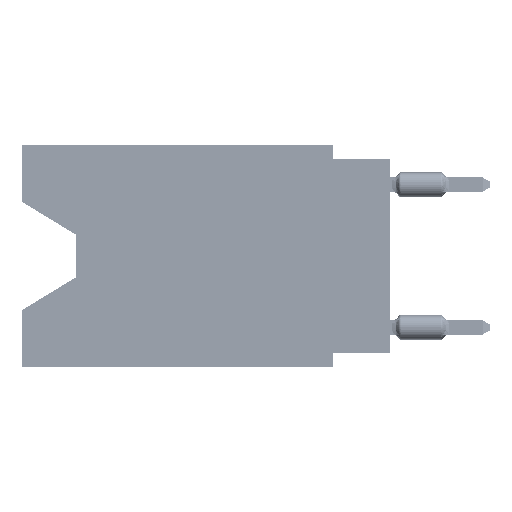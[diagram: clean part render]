
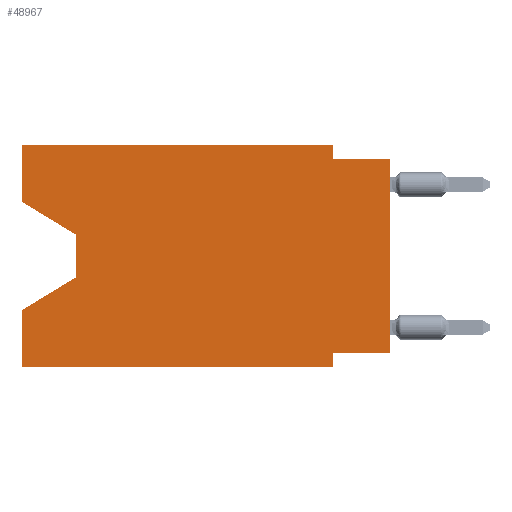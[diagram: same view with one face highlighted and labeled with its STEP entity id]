
A CAD part, left-side view. The second image highlights one B-rep face of the part: STEP entity #48967.
In plain terms, the highlighted planar face has unit normal (-1, 0, 0).
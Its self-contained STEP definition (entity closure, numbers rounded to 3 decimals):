
#384 = EDGE_CURVE ( 'NONE', #65976, #65730, #19403, .T. ) ;
#925 = DIRECTION ( 'NONE',  ( 0., 0., 1. ) ) ;
#1630 = LINE ( 'NONE', #21881, #24821 ) ;
#2386 = ORIENTED_EDGE ( 'NONE', *, *, #59878, .F. ) ;
#3034 = EDGE_CURVE ( 'NONE', #25149, #25658, #43328, .T. ) ;
#4413 = CARTESIAN_POINT ( 'NONE',  ( 0., 16.383, -2.546 ) ) ;
#4581 = LINE ( 'NONE', #29828, #42980 ) ;
#5209 = VECTOR ( 'NONE', #25772, 1000. ) ;
#5611 = ORIENTED_EDGE ( 'NONE', *, *, #67015, .T. ) ;
#5755 = ORIENTED_EDGE ( 'NONE', *, *, #31479, .T. ) ;
#6638 = DIRECTION ( 'NONE',  ( 0., 0., -1. ) ) ;
#7127 = CARTESIAN_POINT ( 'NONE',  ( 0., 16.383, 0. ) ) ;
#7398 = ORIENTED_EDGE ( 'NONE', *, *, #20779, .F. ) ;
#9012 = VECTOR ( 'NONE', #29180, 1000. ) ;
#9027 = ORIENTED_EDGE ( 'NONE', *, *, #65738, .F. ) ;
#9555 = DIRECTION ( 'NONE',  ( 0., -1., 0. ) ) ;
#11085 = VECTOR ( 'NONE', #25171, 1000. ) ;
#13468 = EDGE_LOOP ( 'NONE', ( #39283, #5611, #14471, #36393, #50092, #57030, #2386, #5755, #9027, #33140, #7398, #24245 ) ) ;
#14422 = CARTESIAN_POINT ( 'NONE',  ( 0., 16.383, -9.906 ) ) ;
#14471 = ORIENTED_EDGE ( 'NONE', *, *, #19290, .T. ) ;
#15254 = AXIS2_PLACEMENT_3D ( 'NONE', #66269, #39797, #47651 ) ;
#15755 = CARTESIAN_POINT ( 'NONE',  ( 0., 13.97, -4.013 ) ) ;
#19283 = VECTOR ( 'NONE', #70309, 1000. ) ;
#19290 = EDGE_CURVE ( 'NONE', #57836, #50094, #39008, .T. ) ;
#19403 = LINE ( 'NONE', #20606, #19283 ) ;
#20059 = CARTESIAN_POINT ( 'NONE',  ( 0., 16.383, 0. ) ) ;
#20606 = CARTESIAN_POINT ( 'NONE',  ( 0., 16.383, -9.906 ) ) ;
#20779 = EDGE_CURVE ( 'NONE', #68267, #77958, #39117, .T. ) ;
#21881 = CARTESIAN_POINT ( 'NONE',  ( 0., 2.54, 0. ) ) ;
#24180 = CARTESIAN_POINT ( 'NONE',  ( 0., 2.54, -9.906 ) ) ;
#24245 = ORIENTED_EDGE ( 'NONE', *, *, #66612, .F. ) ;
#24821 = VECTOR ( 'NONE', #40944, 1000. ) ;
#25149 = VERTEX_POINT ( 'NONE', #68659 ) ;
#25171 = DIRECTION ( 'NONE',  ( 0., 0., 1. ) ) ;
#25658 = VERTEX_POINT ( 'NONE', #15755 ) ;
#25772 = DIRECTION ( 'NONE',  ( 0., 0.855, -0.519 ) ) ;
#26176 = CARTESIAN_POINT ( 'NONE',  ( 0., 13.97, -5.893 ) ) ;
#27499 = DIRECTION ( 'NONE',  ( 0., -1., 0. ) ) ;
#29180 = DIRECTION ( 'NONE',  ( 0., 1., 0. ) ) ;
#29828 = CARTESIAN_POINT ( 'NONE',  ( 0., 0., -0.635 ) ) ;
#30149 = LINE ( 'NONE', #70257, #11085 ) ;
#30884 = DIRECTION ( 'NONE',  ( 0., -0.855, -0.519 ) ) ;
#31161 = LINE ( 'NONE', #44004, #62696 ) ;
#31479 = EDGE_CURVE ( 'NONE', #47112, #69940, #30149, .T. ) ;
#33140 = ORIENTED_EDGE ( 'NONE', *, *, #80087, .F. ) ;
#33151 = FACE_OUTER_BOUND ( 'NONE', #13468, .T. ) ;
#36393 = ORIENTED_EDGE ( 'NONE', *, *, #79502, .F. ) ;
#37685 = CARTESIAN_POINT ( 'NONE',  ( 0., 13.97, -4.013 ) ) ;
#39008 = LINE ( 'NONE', #26176, #5209 ) ;
#39117 = LINE ( 'NONE', #20059, #44811 ) ;
#39283 = ORIENTED_EDGE ( 'NONE', *, *, #3034, .T. ) ;
#39797 = DIRECTION ( 'NONE',  ( 1., 0., 0. ) ) ;
#40202 = CARTESIAN_POINT ( 'NONE',  ( 0., 2.54, -0.635 ) ) ;
#40635 = CARTESIAN_POINT ( 'NONE',  ( 0., 13.97, -5.893 ) ) ;
#40944 = DIRECTION ( 'NONE',  ( 0., 0., -1. ) ) ;
#41622 = CARTESIAN_POINT ( 'NONE',  ( 0., 0., -9.271 ) ) ;
#41960 = VECTOR ( 'NONE', #925, 1000. ) ;
#42980 = VECTOR ( 'NONE', #9555, 1000. ) ;
#43328 = LINE ( 'NONE', #4413, #48647 ) ;
#43996 = VECTOR ( 'NONE', #49455, 1000. ) ;
#44004 = CARTESIAN_POINT ( 'NONE',  ( 0., 16.383, 0. ) ) ;
#44811 = VECTOR ( 'NONE', #27499, 1000. ) ;
#45052 = CARTESIAN_POINT ( 'NONE',  ( 0., 16.383, 0. ) ) ;
#47112 = VERTEX_POINT ( 'NONE', #62544 ) ;
#47651 = DIRECTION ( 'NONE',  ( 0., 0., -1. ) ) ;
#48647 = VECTOR ( 'NONE', #30884, 1000. ) ;
#48967 = ADVANCED_FACE ( 'NONE', ( #33151 ), #58420, .F. ) ;
#49046 = VERTEX_POINT ( 'NONE', #40202 ) ;
#49455 = DIRECTION ( 'NONE',  ( 0., 0., -1. ) ) ;
#50092 = ORIENTED_EDGE ( 'NONE', *, *, #384, .T. ) ;
#50094 = VERTEX_POINT ( 'NONE', #57008 ) ;
#56422 = LINE ( 'NONE', #7127, #41960 ) ;
#56845 = DIRECTION ( 'NONE',  ( 0., 0., 1. ) ) ;
#57008 = CARTESIAN_POINT ( 'NONE',  ( 0., 16.383, -7.36 ) ) ;
#57030 = ORIENTED_EDGE ( 'NONE', *, *, #70256, .F. ) ;
#57836 = VERTEX_POINT ( 'NONE', #40635 ) ;
#58420 = PLANE ( 'NONE',  #15254 ) ;
#59878 = EDGE_CURVE ( 'NONE', #47112, #79579, #73912, .T. ) ;
#62544 = CARTESIAN_POINT ( 'NONE',  ( 0., 0., -9.271 ) ) ;
#62696 = VECTOR ( 'NONE', #56845, 1000. ) ;
#65730 = VERTEX_POINT ( 'NONE', #67509 ) ;
#65738 = EDGE_CURVE ( 'NONE', #49046, #69940, #4581, .T. ) ;
#65976 = VERTEX_POINT ( 'NONE', #14422 ) ;
#66269 = CARTESIAN_POINT ( 'NONE',  ( 0., 16.383, 0. ) ) ;
#66612 = EDGE_CURVE ( 'NONE', #25149, #68267, #31161, .T. ) ;
#67015 = EDGE_CURVE ( 'NONE', #25658, #57836, #68742, .T. ) ;
#67509 = CARTESIAN_POINT ( 'NONE',  ( 0., 2.54, -9.906 ) ) ;
#68267 = VERTEX_POINT ( 'NONE', #45052 ) ;
#68659 = CARTESIAN_POINT ( 'NONE',  ( 0., 16.383, -2.546 ) ) ;
#68742 = LINE ( 'NONE', #37685, #71974 ) ;
#69940 = VERTEX_POINT ( 'NONE', #70190 ) ;
#70049 = CARTESIAN_POINT ( 'NONE',  ( 0., 2.54, -9.271 ) ) ;
#70190 = CARTESIAN_POINT ( 'NONE',  ( 0., 0., -0.635 ) ) ;
#70256 = EDGE_CURVE ( 'NONE', #79579, #65730, #80909, .T. ) ;
#70257 = CARTESIAN_POINT ( 'NONE',  ( 0., 0., 0. ) ) ;
#70309 = DIRECTION ( 'NONE',  ( 0., -1., 0. ) ) ;
#71882 = CARTESIAN_POINT ( 'NONE',  ( 0., 2.54, 0. ) ) ;
#71974 = VECTOR ( 'NONE', #6638, 1000. ) ;
#73912 = LINE ( 'NONE', #41622, #9012 ) ;
#77958 = VERTEX_POINT ( 'NONE', #71882 ) ;
#79502 = EDGE_CURVE ( 'NONE', #65976, #50094, #56422, .T. ) ;
#79579 = VERTEX_POINT ( 'NONE', #70049 ) ;
#80087 = EDGE_CURVE ( 'NONE', #77958, #49046, #1630, .T. ) ;
#80909 = LINE ( 'NONE', #24180, #43996 ) ;
